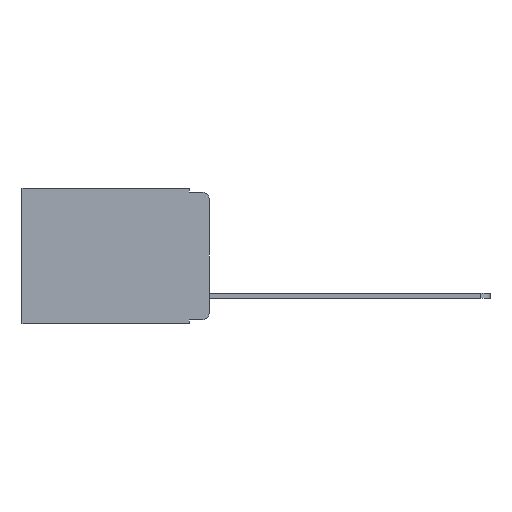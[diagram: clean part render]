
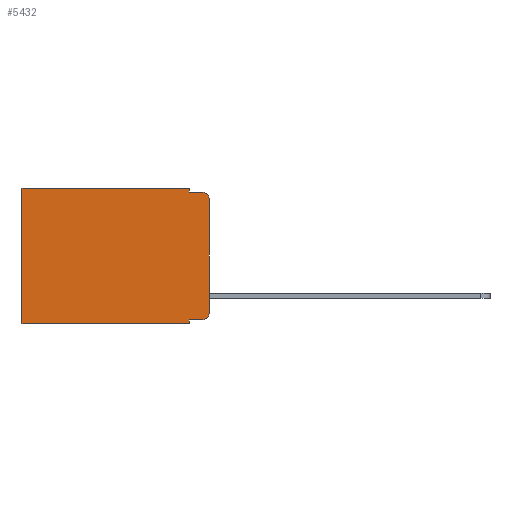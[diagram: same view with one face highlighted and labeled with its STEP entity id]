
A CAD part, left-side view. The second image highlights one B-rep face of the part: STEP entity #5432.
In plain terms, the highlighted planar face has unit normal (-1, 0, 0).
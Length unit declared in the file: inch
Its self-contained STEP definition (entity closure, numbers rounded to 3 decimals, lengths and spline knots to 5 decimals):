
#215 = EDGE_CURVE ( 'NONE', #3410, #8105, #2750, .T. ) ;
#251 = LINE ( 'NONE', #7242, #2934 ) ;
#333 = VECTOR ( 'NONE', #7428, 39.37008 ) ;
#354 = ORIENTED_EDGE ( 'NONE', *, *, #4163, .F. ) ;
#613 = ORIENTED_EDGE ( 'NONE', *, *, #9545, .T. ) ;
#730 = VECTOR ( 'NONE', #10804, 39.37008 ) ;
#736 = DIRECTION ( 'NONE',  ( 0., 0., -1. ) ) ;
#954 = CARTESIAN_POINT ( 'NONE',  ( 0.298, 0.051, 0. ) ) ;
#958 = CARTESIAN_POINT ( 'NONE',  ( 0.298, 0., -0.313 ) ) ;
#1104 = VERTEX_POINT ( 'NONE', #3498 ) ;
#1139 = VECTOR ( 'NONE', #6180, 39.37008 ) ;
#1147 = ORIENTED_EDGE ( 'NONE', *, *, #4931, .T. ) ;
#1362 = VERTEX_POINT ( 'NONE', #10898 ) ;
#1375 = ORIENTED_EDGE ( 'NONE', *, *, #6675, .F. ) ;
#1690 = VECTOR ( 'NONE', #6551, 39.37008 ) ;
#1715 = AXIS2_PLACEMENT_3D ( 'NONE', #9785, #10801, #5529 ) ;
#1865 = VERTEX_POINT ( 'NONE', #1941 ) ;
#1941 = CARTESIAN_POINT ( 'NONE',  ( 0.298, 0.051, -0.343 ) ) ;
#2167 = DIRECTION ( 'NONE',  ( 0., 0., -1. ) ) ;
#2329 = ORIENTED_EDGE ( 'NONE', *, *, #2853, .F. ) ;
#2358 = CIRCLE ( 'NONE', #2661, 0.02 ) ;
#2661 = AXIS2_PLACEMENT_3D ( 'NONE', #5178, #10870, #6051 ) ;
#2750 = LINE ( 'NONE', #10446, #333 ) ;
#2801 = ORIENTED_EDGE ( 'NONE', *, *, #10067, .T. ) ;
#2833 = VECTOR ( 'NONE', #2167, 39.37008 ) ;
#2853 = EDGE_CURVE ( 'NONE', #5576, #7652, #5430, .T. ) ;
#2934 = VECTOR ( 'NONE', #3785, 39.37008 ) ;
#3040 = CARTESIAN_POINT ( 'NONE',  ( 0.298, 0.051, 0. ) ) ;
#3055 = CIRCLE ( 'NONE', #1715, 0.02 ) ;
#3171 = VERTEX_POINT ( 'NONE', #6618 ) ;
#3330 = VECTOR ( 'NONE', #8250, 39.37008 ) ;
#3333 = CARTESIAN_POINT ( 'NONE',  ( 0.298, 0., -0.343 ) ) ;
#3410 = VERTEX_POINT ( 'NONE', #954 ) ;
#3498 = CARTESIAN_POINT ( 'NONE',  ( 0.298, 0.02, -0.333 ) ) ;
#3730 = VECTOR ( 'NONE', #736, 39.37008 ) ;
#3785 = DIRECTION ( 'NONE',  ( 0., -1., 0. ) ) ;
#4163 = EDGE_CURVE ( 'NONE', #1865, #1362, #5937, .T. ) ;
#4216 = ORIENTED_EDGE ( 'NONE', *, *, #8493, .F. ) ;
#4233 = ORIENTED_EDGE ( 'NONE', *, *, #5525, .T. ) ;
#4429 = CARTESIAN_POINT ( 'NONE',  ( 0.298, 0.051, -0.333 ) ) ;
#4475 = VERTEX_POINT ( 'NONE', #7064 ) ;
#4495 = ORIENTED_EDGE ( 'NONE', *, *, #7787, .F. ) ;
#4556 = FACE_OUTER_BOUND ( 'NONE', #8138, .T. ) ;
#4596 = CARTESIAN_POINT ( 'NONE',  ( 0.298, 0., 0. ) ) ;
#4931 = EDGE_CURVE ( 'NONE', #5576, #10789, #3055, .T. ) ;
#5178 = CARTESIAN_POINT ( 'NONE',  ( 0.298, 0.02, -0.313 ) ) ;
#5212 = CARTESIAN_POINT ( 'NONE',  ( 0.298, 0.473, 0. ) ) ;
#5430 = LINE ( 'NONE', #10012, #730 ) ;
#5432 = ADVANCED_FACE ( 'NONE', ( #4556 ), #7638, .F. ) ;
#5525 = EDGE_CURVE ( 'NONE', #8105, #1362, #6053, .T. ) ;
#5529 = DIRECTION ( 'NONE',  ( 0., 0., -1. ) ) ;
#5557 = DIRECTION ( 'NONE',  ( 1., 0., 0. ) ) ;
#5576 = VERTEX_POINT ( 'NONE', #9538 ) ;
#5778 = LINE ( 'NONE', #4429, #1139 ) ;
#5937 = LINE ( 'NONE', #3333, #3330 ) ;
#6051 = DIRECTION ( 'NONE',  ( 0., 0., -1. ) ) ;
#6053 = LINE ( 'NONE', #5212, #3730 ) ;
#6126 = DIRECTION ( 'NONE',  ( 0., 0., -1. ) ) ;
#6155 = CARTESIAN_POINT ( 'NONE',  ( 0.298, 0.02, -0.01 ) ) ;
#6180 = DIRECTION ( 'NONE',  ( 0., -1., 0. ) ) ;
#6339 = LINE ( 'NONE', #3040, #1690 ) ;
#6551 = DIRECTION ( 'NONE',  ( 0., 0., -1. ) ) ;
#6618 = CARTESIAN_POINT ( 'NONE',  ( 0.298, 0.051, -0.01 ) ) ;
#6675 = EDGE_CURVE ( 'NONE', #3410, #3171, #7186, .T. ) ;
#7064 = CARTESIAN_POINT ( 'NONE',  ( 0.298, 0.051, -0.333 ) ) ;
#7186 = LINE ( 'NONE', #7369, #2833 ) ;
#7242 = CARTESIAN_POINT ( 'NONE',  ( 0.298, 0.051, -0.01 ) ) ;
#7369 = CARTESIAN_POINT ( 'NONE',  ( 0.298, 0.051, 0. ) ) ;
#7428 = DIRECTION ( 'NONE',  ( 0., 1., 0. ) ) ;
#7497 = ORIENTED_EDGE ( 'NONE', *, *, #215, .T. ) ;
#7638 = PLANE ( 'NONE',  #8913 ) ;
#7652 = VERTEX_POINT ( 'NONE', #958 ) ;
#7787 = EDGE_CURVE ( 'NONE', #3171, #10789, #251, .T. ) ;
#8105 = VERTEX_POINT ( 'NONE', #10784 ) ;
#8138 = EDGE_LOOP ( 'NONE', ( #2329, #1147, #4495, #1375, #7497, #4233, #354, #4216, #613, #2801 ) ) ;
#8250 = DIRECTION ( 'NONE',  ( 0., 1., 0. ) ) ;
#8493 = EDGE_CURVE ( 'NONE', #4475, #1865, #6339, .T. ) ;
#8913 = AXIS2_PLACEMENT_3D ( 'NONE', #4596, #5557, #6126 ) ;
#9538 = CARTESIAN_POINT ( 'NONE',  ( 0.298, 0., -0.03 ) ) ;
#9545 = EDGE_CURVE ( 'NONE', #4475, #1104, #5778, .T. ) ;
#9785 = CARTESIAN_POINT ( 'NONE',  ( 0.298, 0.02, -0.03 ) ) ;
#10012 = CARTESIAN_POINT ( 'NONE',  ( 0.298, 0., 0. ) ) ;
#10067 = EDGE_CURVE ( 'NONE', #1104, #7652, #2358, .T. ) ;
#10446 = CARTESIAN_POINT ( 'NONE',  ( 0.298, 0., 0. ) ) ;
#10784 = CARTESIAN_POINT ( 'NONE',  ( 0.298, 0.473, 0. ) ) ;
#10789 = VERTEX_POINT ( 'NONE', #6155 ) ;
#10801 = DIRECTION ( 'NONE',  ( -1., 0., 0. ) ) ;
#10804 = DIRECTION ( 'NONE',  ( 0., 0., -1. ) ) ;
#10870 = DIRECTION ( 'NONE',  ( -1., 0., 0. ) ) ;
#10898 = CARTESIAN_POINT ( 'NONE',  ( 0.298, 0.473, -0.343 ) ) ;
